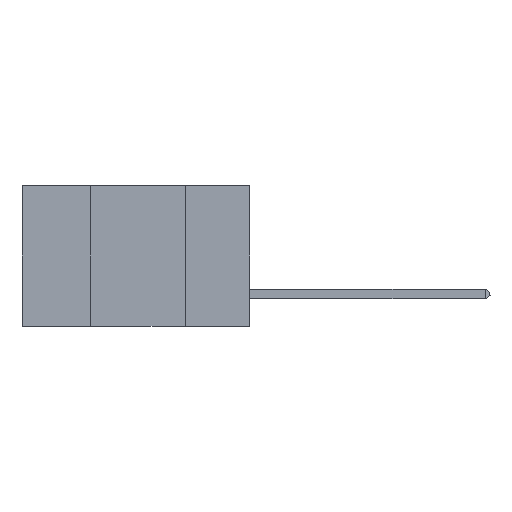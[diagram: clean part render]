
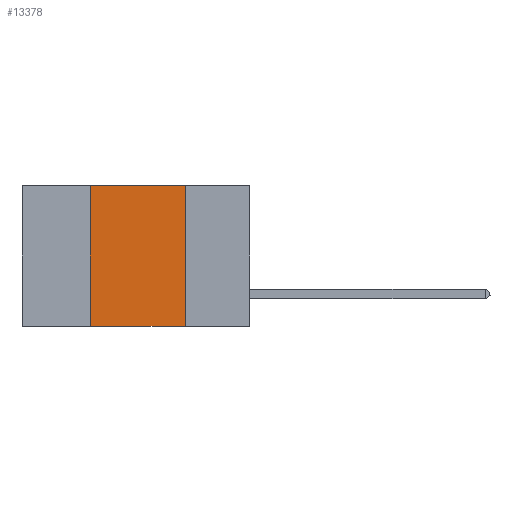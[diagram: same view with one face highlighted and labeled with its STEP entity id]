
A CAD part, left-side view. The second image highlights one B-rep face of the part: STEP entity #13378.
In plain terms, the highlighted planar face has unit normal (-1, 0, 0).
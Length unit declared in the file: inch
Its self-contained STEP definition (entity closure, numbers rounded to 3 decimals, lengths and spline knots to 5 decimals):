
#638 = ORIENTED_EDGE ( 'NONE', *, *, #13461, .T. ) ;
#799 = VECTOR ( 'NONE', #10536, 39.37008 ) ;
#2222 = CARTESIAN_POINT ( 'NONE',  ( 0., 0.17, 0. ) ) ;
#2645 = CARTESIAN_POINT ( 'NONE',  ( 0., 0.42, -0.37 ) ) ;
#4260 = CARTESIAN_POINT ( 'NONE',  ( 0., 0.42, 0. ) ) ;
#4318 = EDGE_LOOP ( 'NONE', ( #5633, #11071, #9897, #638 ) ) ;
#4340 = VERTEX_POINT ( 'NONE', #4260 ) ;
#5101 = CARTESIAN_POINT ( 'NONE',  ( 0., 0.17, 0. ) ) ;
#5212 = EDGE_CURVE ( 'NONE', #7830, #12105, #9054, .T. ) ;
#5269 = AXIS2_PLACEMENT_3D ( 'NONE', #9506, #9547, #12640 ) ;
#5444 = VECTOR ( 'NONE', #12593, 39.37008 ) ;
#5633 = ORIENTED_EDGE ( 'NONE', *, *, #5212, .F. ) ;
#6431 = LINE ( 'NONE', #6624, #9337 ) ;
#6624 = CARTESIAN_POINT ( 'NONE',  ( 0., 0.6, -0.37 ) ) ;
#7064 = LINE ( 'NONE', #7980, #12553 ) ;
#7478 = CARTESIAN_POINT ( 'NONE',  ( 0., 0.42, 0. ) ) ;
#7830 = VERTEX_POINT ( 'NONE', #5101 ) ;
#7980 = CARTESIAN_POINT ( 'NONE',  ( 0., 0.6, 0. ) ) ;
#8414 = PLANE ( 'NONE',  #5269 ) ;
#8493 = LINE ( 'NONE', #7478, #799 ) ;
#8713 = EDGE_CURVE ( 'NONE', #10768, #4340, #8493, .T. ) ;
#9054 = LINE ( 'NONE', #2222, #5444 ) ;
#9294 = DIRECTION ( 'NONE',  ( 0., -1., 0. ) ) ;
#9337 = VECTOR ( 'NONE', #9294, 39.37008 ) ;
#9506 = CARTESIAN_POINT ( 'NONE',  ( 0., 0.6, 0. ) ) ;
#9547 = DIRECTION ( 'NONE',  ( 1., 0., 0. ) ) ;
#9897 = ORIENTED_EDGE ( 'NONE', *, *, #8713, .F. ) ;
#10536 = DIRECTION ( 'NONE',  ( 0., 0., 1. ) ) ;
#10768 = VERTEX_POINT ( 'NONE', #2645 ) ;
#11021 = FACE_OUTER_BOUND ( 'NONE', #4318, .T. ) ;
#11071 = ORIENTED_EDGE ( 'NONE', *, *, #12374, .F. ) ;
#11150 = DIRECTION ( 'NONE',  ( 0., -1., 0. ) ) ;
#12105 = VERTEX_POINT ( 'NONE', #13772 ) ;
#12374 = EDGE_CURVE ( 'NONE', #4340, #7830, #7064, .T. ) ;
#12553 = VECTOR ( 'NONE', #11150, 39.37008 ) ;
#12593 = DIRECTION ( 'NONE',  ( 0., 0., -1. ) ) ;
#12640 = DIRECTION ( 'NONE',  ( 0., 0., -1. ) ) ;
#13378 = ADVANCED_FACE ( 'NONE', ( #11021 ), #8414, .F. ) ;
#13461 = EDGE_CURVE ( 'NONE', #10768, #12105, #6431, .T. ) ;
#13772 = CARTESIAN_POINT ( 'NONE',  ( 0., 0.17, -0.37 ) ) ;
